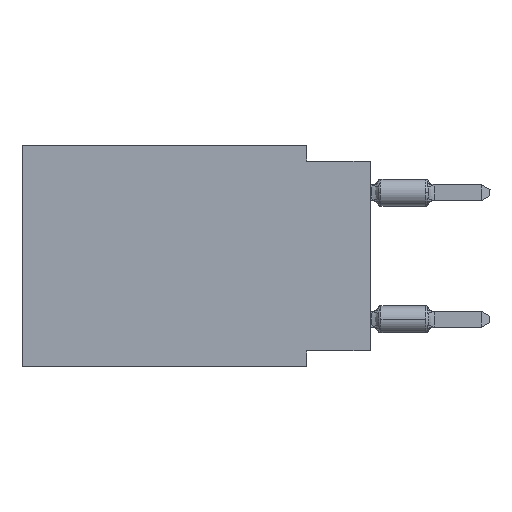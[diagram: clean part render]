
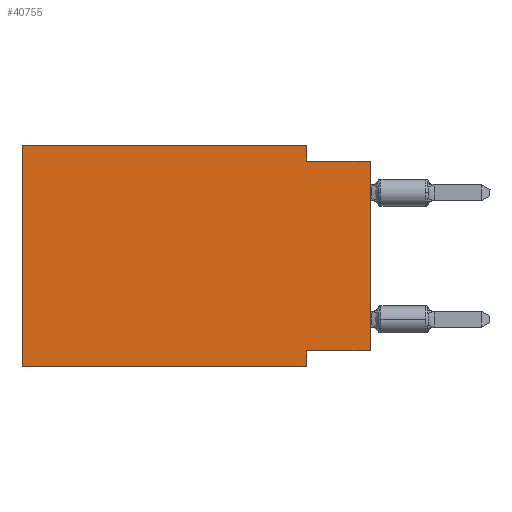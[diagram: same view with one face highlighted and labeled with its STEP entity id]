
A CAD part, left-side view. The second image highlights one B-rep face of the part: STEP entity #40755.
In plain terms, the highlighted planar face has unit normal (-1, 0, 0).
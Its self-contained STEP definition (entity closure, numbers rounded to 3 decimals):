
#268 = DIRECTION ( 'NONE',  ( 0., 0., -1. ) ) ;
#971 = CARTESIAN_POINT ( 'NONE',  ( 0., 0., 0. ) ) ;
#1504 = EDGE_CURVE ( 'NONE', #5884, #32801, #35796, .T. ) ;
#1648 = VECTOR ( 'NONE', #40617, 1000. ) ;
#2508 = ORIENTED_EDGE ( 'NONE', *, *, #15469, .F. ) ;
#2921 = CARTESIAN_POINT ( 'NONE',  ( 0., 2.54, -0.635 ) ) ;
#3873 = AXIS2_PLACEMENT_3D ( 'NONE', #27567, #45670, #268 ) ;
#3915 = EDGE_CURVE ( 'NONE', #5884, #5471, #55981, .T. ) ;
#3930 = CARTESIAN_POINT ( 'NONE',  ( 0., 0., -0.635 ) ) ;
#4281 = CARTESIAN_POINT ( 'NONE',  ( 0., 0., -8.255 ) ) ;
#5183 = ORIENTED_EDGE ( 'NONE', *, *, #3915, .T. ) ;
#5471 = VERTEX_POINT ( 'NONE', #20204 ) ;
#5539 = DIRECTION ( 'NONE',  ( 0., -1., 0. ) ) ;
#5884 = VERTEX_POINT ( 'NONE', #4281 ) ;
#6986 = DIRECTION ( 'NONE',  ( 0., 0., -1. ) ) ;
#7381 = DIRECTION ( 'NONE',  ( 0., 0., 1. ) ) ;
#7498 = EDGE_CURVE ( 'NONE', #39882, #5471, #58899, .T. ) ;
#9408 = VERTEX_POINT ( 'NONE', #14525 ) ;
#9732 = EDGE_LOOP ( 'NONE', ( #5183, #44658, #42561, #12680, #43506, #18023, #2508, #34275 ) ) ;
#11226 = CARTESIAN_POINT ( 'NONE',  ( 0., 2.54, -8.255 ) ) ;
#12680 = ORIENTED_EDGE ( 'NONE', *, *, #15260, .F. ) ;
#13513 = VECTOR ( 'NONE', #22208, 1000. ) ;
#14500 = CARTESIAN_POINT ( 'NONE',  ( 0., 13.97, 0. ) ) ;
#14525 = CARTESIAN_POINT ( 'NONE',  ( 0., 2.54, -8.89 ) ) ;
#14748 = DIRECTION ( 'NONE',  ( 0., 0., 1. ) ) ;
#15260 = EDGE_CURVE ( 'NONE', #38182, #31802, #46419, .T. ) ;
#15275 = DIRECTION ( 'NONE',  ( 0., 0., -1. ) ) ;
#15469 = EDGE_CURVE ( 'NONE', #32801, #9408, #42665, .T. ) ;
#16265 = EDGE_CURVE ( 'NONE', #31802, #39882, #56580, .T. ) ;
#18023 = ORIENTED_EDGE ( 'NONE', *, *, #31556, .T. ) ;
#19295 = VECTOR ( 'NONE', #54837, 1000. ) ;
#19408 = VERTEX_POINT ( 'NONE', #22382 ) ;
#20204 = CARTESIAN_POINT ( 'NONE',  ( 0., 0., -0.635 ) ) ;
#22208 = DIRECTION ( 'NONE',  ( 0., -1., 0. ) ) ;
#22382 = CARTESIAN_POINT ( 'NONE',  ( 0., 13.97, -8.89 ) ) ;
#24699 = CARTESIAN_POINT ( 'NONE',  ( 0., 13.97, -8.89 ) ) ;
#26272 = LINE ( 'NONE', #30492, #39569 ) ;
#27280 = PLANE ( 'NONE',  #3873 ) ;
#27567 = CARTESIAN_POINT ( 'NONE',  ( 0., 13.97, 0. ) ) ;
#30492 = CARTESIAN_POINT ( 'NONE',  ( 0., 13.97, 0. ) ) ;
#31239 = EDGE_CURVE ( 'NONE', #19408, #38182, #26272, .T. ) ;
#31556 = EDGE_CURVE ( 'NONE', #19408, #9408, #56616, .T. ) ;
#31802 = VERTEX_POINT ( 'NONE', #50495 ) ;
#32801 = VERTEX_POINT ( 'NONE', #11226 ) ;
#33405 = CARTESIAN_POINT ( 'NONE',  ( 0., 2.54, 0. ) ) ;
#34275 = ORIENTED_EDGE ( 'NONE', *, *, #1504, .F. ) ;
#35191 = CARTESIAN_POINT ( 'NONE',  ( 0., 0., -8.255 ) ) ;
#35796 = LINE ( 'NONE', #35191, #1648 ) ;
#38182 = VERTEX_POINT ( 'NONE', #53967 ) ;
#39569 = VECTOR ( 'NONE', #7381, 1000. ) ;
#39577 = CARTESIAN_POINT ( 'NONE',  ( 0., 2.54, -8.89 ) ) ;
#39882 = VERTEX_POINT ( 'NONE', #2921 ) ;
#40617 = DIRECTION ( 'NONE',  ( 0., 1., 0. ) ) ;
#40755 = ADVANCED_FACE ( 'NONE', ( #50469 ), #27280, .F. ) ;
#42194 = VECTOR ( 'NONE', #14748, 1000. ) ;
#42561 = ORIENTED_EDGE ( 'NONE', *, *, #16265, .F. ) ;
#42665 = LINE ( 'NONE', #39577, #56795 ) ;
#43506 = ORIENTED_EDGE ( 'NONE', *, *, #31239, .F. ) ;
#44658 = ORIENTED_EDGE ( 'NONE', *, *, #7498, .F. ) ;
#45670 = DIRECTION ( 'NONE',  ( 1., 0., 0. ) ) ;
#46419 = LINE ( 'NONE', #14500, #19295 ) ;
#50469 = FACE_OUTER_BOUND ( 'NONE', #9732, .T. ) ;
#50495 = CARTESIAN_POINT ( 'NONE',  ( 0., 2.54, 0. ) ) ;
#53967 = CARTESIAN_POINT ( 'NONE',  ( 0., 13.97, 0. ) ) ;
#54837 = DIRECTION ( 'NONE',  ( 0., -1., 0. ) ) ;
#54961 = VECTOR ( 'NONE', #6986, 1000. ) ;
#55981 = LINE ( 'NONE', #971, #42194 ) ;
#56580 = LINE ( 'NONE', #33405, #54961 ) ;
#56616 = LINE ( 'NONE', #24699, #58813 ) ;
#56795 = VECTOR ( 'NONE', #15275, 1000. ) ;
#58813 = VECTOR ( 'NONE', #5539, 1000. ) ;
#58899 = LINE ( 'NONE', #3930, #13513 ) ;
